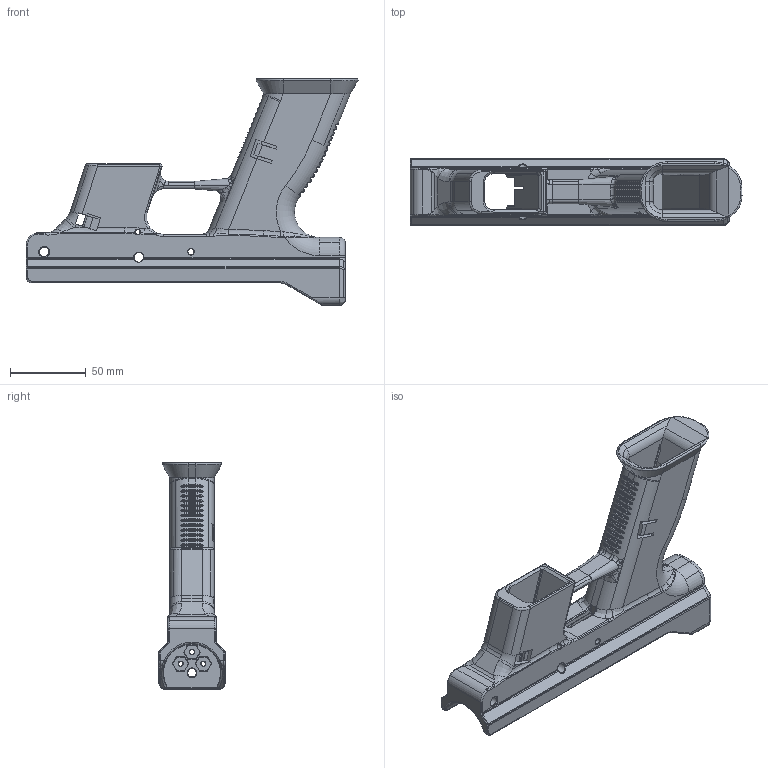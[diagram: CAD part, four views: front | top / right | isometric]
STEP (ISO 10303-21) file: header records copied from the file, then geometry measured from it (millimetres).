
FILE_DESCRIPTION (( 'STEP AP203' ), '1' );
FILE_NAME ('GAB-10_V3.STEP', '2020-02-07T01:26:00', ( '' ), ( '' ), 'SwSTEP 2.0', 'SolidWorks 2019', '' );
FILE_SCHEMA (( 'CONFIG_CONTROL_DESIGN' ));
Products named in the file (1): GAB-10_V3
Bounding box: 219.35 x 44 x 149.96 mm (x, y, z)
Volume: 240927.2 mm3; surface area: 83856.4 mm2
Topology: 1 solids, 1 shells, 1231 faces, 3134 edges, 1865 vertices
Faces by surface type: cylinder 477, bspline 389, plane 238, torus 75, cone 50, sphere 2
Entity records: 52882 total; most frequent: CARTESIAN_POINT 27365, ORIENTED_EDGE 6216, DIRECTION 3838, EDGE_CURVE 3108, VERTEX_POINT 1865, B_SPLINE_CURVE_WITH_KNOTS 1369, AXIS2_PLACEMENT_3D 1367, EDGE_LOOP 1253
